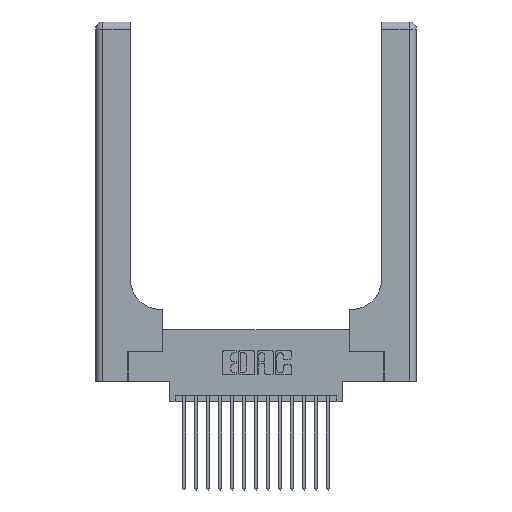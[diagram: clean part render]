
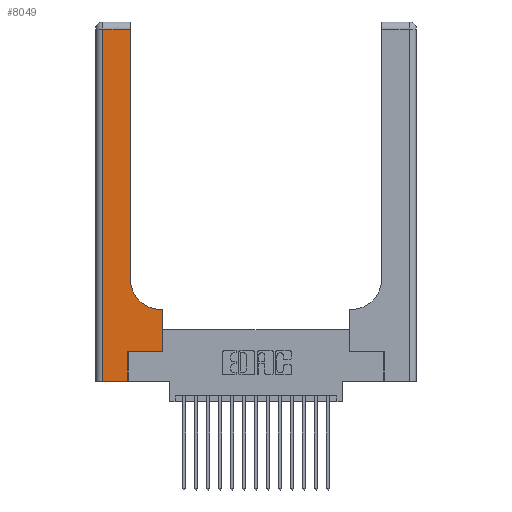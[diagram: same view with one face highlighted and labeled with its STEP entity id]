
A CAD part, top view. The second image highlights one B-rep face of the part: STEP entity #8049.
In plain terms, the highlighted planar face has unit normal (0, 0, 1).
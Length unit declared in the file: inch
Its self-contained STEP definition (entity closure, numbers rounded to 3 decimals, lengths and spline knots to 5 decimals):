
#467 = CARTESIAN_POINT ( 'NONE',  ( 0.5415, 0.6, 0.37 ) ) ;
#553 = CIRCLE ( 'NONE', #11683, 0.25 ) ;
#615 = EDGE_LOOP ( 'NONE', ( #773, #12882, #755, #3181, #16998, #7289, #19259, #2209, #10323 ) ) ;
#729 = VECTOR ( 'NONE', #8501, 39.37008 ) ;
#755 = ORIENTED_EDGE ( 'NONE', *, *, #2791, .T. ) ;
#773 = ORIENTED_EDGE ( 'NONE', *, *, #18563, .T. ) ;
#807 = CARTESIAN_POINT ( 'NONE',  ( 0.06, 0., 0.37 ) ) ;
#1097 = VERTEX_POINT ( 'NONE', #9482 ) ;
#1718 = DIRECTION ( 'NONE',  ( 0., 0., -1. ) ) ;
#2209 = ORIENTED_EDGE ( 'NONE', *, *, #17923, .T. ) ;
#2223 = EDGE_CURVE ( 'NONE', #1097, #6672, #15400, .T. ) ;
#2232 = CARTESIAN_POINT ( 'NONE',  ( 0.5585, 0.25, 0.37 ) ) ;
#2637 = EDGE_CURVE ( 'NONE', #17477, #15336, #12835, .T. ) ;
#2791 = EDGE_CURVE ( 'NONE', #6672, #12981, #17883, .T. ) ;
#3156 = CARTESIAN_POINT ( 'NONE',  ( 0.06, 2.94, 0.37 ) ) ;
#3181 = ORIENTED_EDGE ( 'NONE', *, *, #5027, .T. ) ;
#3278 = CARTESIAN_POINT ( 'NONE',  ( 0.2915, 0.6, 0.37 ) ) ;
#3288 = LINE ( 'NONE', #9156, #10462 ) ;
#4257 = CARTESIAN_POINT ( 'NONE',  ( 0.06, 3., 0.37 ) ) ;
#5027 = EDGE_CURVE ( 'NONE', #12981, #16667, #7071, .T. ) ;
#6109 = DIRECTION ( 'NONE',  ( 0., 1., 0. ) ) ;
#6127 = CARTESIAN_POINT ( 'NONE',  ( 0.5585, 0.25, 0.37 ) ) ;
#6567 = VECTOR ( 'NONE', #13246, 39.37008 ) ;
#6672 = VERTEX_POINT ( 'NONE', #3156 ) ;
#6769 = CARTESIAN_POINT ( 'NONE',  ( 0., 3., 0.37 ) ) ;
#7071 = LINE ( 'NONE', #13902, #18353 ) ;
#7289 = ORIENTED_EDGE ( 'NONE', *, *, #2637, .T. ) ;
#7397 = CARTESIAN_POINT ( 'NONE',  ( 0., 2.94, 0.37 ) ) ;
#7738 = EDGE_CURVE ( 'NONE', #15336, #9127, #14148, .T. ) ;
#7954 = DIRECTION ( 'NONE',  ( -1., 0., 0. ) ) ;
#8018 = VECTOR ( 'NONE', #8932, 39.37008 ) ;
#8049 = ADVANCED_FACE ( 'NONE', ( #16862 ), #11210, .F. ) ;
#8292 = DIRECTION ( 'NONE',  ( 0., 0., -1. ) ) ;
#8501 = DIRECTION ( 'NONE',  ( 1., 0., 0. ) ) ;
#8660 = VERTEX_POINT ( 'NONE', #16871 ) ;
#8932 = DIRECTION ( 'NONE',  ( -1., 0., 0. ) ) ;
#9127 = VERTEX_POINT ( 'NONE', #12503 ) ;
#9156 = CARTESIAN_POINT ( 'NONE',  ( 0.269, 0., 0.37 ) ) ;
#9482 = CARTESIAN_POINT ( 'NONE',  ( 0.2915, 2.94, 0.37 ) ) ;
#9598 = VECTOR ( 'NONE', #7954, 39.37008 ) ;
#9984 = CARTESIAN_POINT ( 'NONE',  ( 0.269, 0.25, 0.37 ) ) ;
#10058 = LINE ( 'NONE', #3278, #9598 ) ;
#10323 = ORIENTED_EDGE ( 'NONE', *, *, #10431, .T. ) ;
#10431 = EDGE_CURVE ( 'NONE', #18904, #8660, #553, .T. ) ;
#10462 = VECTOR ( 'NONE', #6109, 39.37008 ) ;
#10638 = DIRECTION ( 'NONE',  ( 0., 1., 0. ) ) ;
#10729 = VECTOR ( 'NONE', #17582, 39.37008 ) ;
#10878 = CARTESIAN_POINT ( 'NONE',  ( 0.5415, 0.85, 0.37 ) ) ;
#11210 = PLANE ( 'NONE',  #14973 ) ;
#11683 = AXIS2_PLACEMENT_3D ( 'NONE', #10878, #1718, #12328 ) ;
#12057 = EDGE_CURVE ( 'NONE', #16667, #17477, #3288, .T. ) ;
#12328 = DIRECTION ( 'NONE',  ( 1., 0., 0. ) ) ;
#12503 = CARTESIAN_POINT ( 'NONE',  ( 0.5585, 0.6, 0.37 ) ) ;
#12835 = LINE ( 'NONE', #9984, #729 ) ;
#12882 = ORIENTED_EDGE ( 'NONE', *, *, #2223, .T. ) ;
#12981 = VERTEX_POINT ( 'NONE', #807 ) ;
#13246 = DIRECTION ( 'NONE',  ( 0., -1., 0. ) ) ;
#13692 = VECTOR ( 'NONE', #10638, 39.37008 ) ;
#13902 = CARTESIAN_POINT ( 'NONE',  ( 0., 0., 0.37 ) ) ;
#14148 = LINE ( 'NONE', #6127, #13692 ) ;
#14601 = CARTESIAN_POINT ( 'NONE',  ( 0.2915, 3., 0.37 ) ) ;
#14638 = LINE ( 'NONE', #14601, #10729 ) ;
#14973 = AXIS2_PLACEMENT_3D ( 'NONE', #6769, #8292, #18554 ) ;
#15336 = VERTEX_POINT ( 'NONE', #2232 ) ;
#15400 = LINE ( 'NONE', #7397, #8018 ) ;
#16667 = VERTEX_POINT ( 'NONE', #17767 ) ;
#16830 = DIRECTION ( 'NONE',  ( 1., 0., 0. ) ) ;
#16862 = FACE_OUTER_BOUND ( 'NONE', #615, .T. ) ;
#16871 = CARTESIAN_POINT ( 'NONE',  ( 0.2915, 0.85, 0.37 ) ) ;
#16998 = ORIENTED_EDGE ( 'NONE', *, *, #12057, .T. ) ;
#17477 = VERTEX_POINT ( 'NONE', #18181 ) ;
#17582 = DIRECTION ( 'NONE',  ( 0., 1., 0. ) ) ;
#17767 = CARTESIAN_POINT ( 'NONE',  ( 0.269, 0., 0.37 ) ) ;
#17883 = LINE ( 'NONE', #4257, #6567 ) ;
#17923 = EDGE_CURVE ( 'NONE', #9127, #18904, #10058, .T. ) ;
#18181 = CARTESIAN_POINT ( 'NONE',  ( 0.269, 0.25, 0.37 ) ) ;
#18353 = VECTOR ( 'NONE', #16830, 39.37008 ) ;
#18554 = DIRECTION ( 'NONE',  ( -1., 0., 0. ) ) ;
#18563 = EDGE_CURVE ( 'NONE', #8660, #1097, #14638, .T. ) ;
#18904 = VERTEX_POINT ( 'NONE', #467 ) ;
#19259 = ORIENTED_EDGE ( 'NONE', *, *, #7738, .T. ) ;
